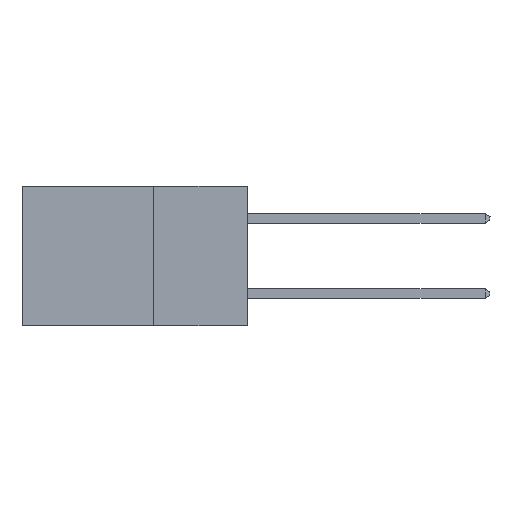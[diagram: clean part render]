
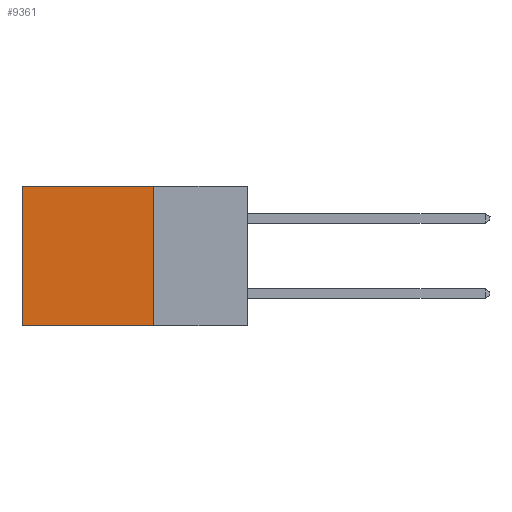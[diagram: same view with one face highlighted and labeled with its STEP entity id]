
A CAD part, left-side view. The second image highlights one B-rep face of the part: STEP entity #9361.
In plain terms, the highlighted planar face has unit normal (-1, 0, 0).
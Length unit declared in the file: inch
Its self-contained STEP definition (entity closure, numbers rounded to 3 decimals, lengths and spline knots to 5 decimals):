
#234 = CARTESIAN_POINT ( 'NONE',  ( 0.298, 0.6, 0. ) ) ;
#791 = VECTOR ( 'NONE', #5980, 39.37008 ) ;
#3077 = DIRECTION ( 'NONE',  ( 1., 0., 0. ) ) ;
#3121 = EDGE_CURVE ( 'NONE', #14947, #22055, #24953, .T. ) ;
#4579 = EDGE_CURVE ( 'NONE', #10231, #8371, #10458, .T. ) ;
#4825 = ORIENTED_EDGE ( 'NONE', *, *, #10721, .F. ) ;
#5660 = CARTESIAN_POINT ( 'NONE',  ( 0.298, 0.6, -0.37 ) ) ;
#5980 = DIRECTION ( 'NONE',  ( 0., 0., -1. ) ) ;
#6827 = VECTOR ( 'NONE', #19081, 39.37008 ) ;
#7606 = EDGE_LOOP ( 'NONE', ( #22664, #16860, #4825, #17059 ) ) ;
#8371 = VERTEX_POINT ( 'NONE', #23700 ) ;
#8498 = VECTOR ( 'NONE', #12989, 39.37008 ) ;
#9361 = ADVANCED_FACE ( 'NONE', ( #17837 ), #17186, .F. ) ;
#10231 = VERTEX_POINT ( 'NONE', #25343 ) ;
#10458 = LINE ( 'NONE', #19895, #18463 ) ;
#10721 = EDGE_CURVE ( 'NONE', #10231, #14947, #19887, .T. ) ;
#12240 = DIRECTION ( 'NONE',  ( 0., 1., 0. ) ) ;
#12634 = CARTESIAN_POINT ( 'NONE',  ( 0.298, 0.25, 0. ) ) ;
#12989 = DIRECTION ( 'NONE',  ( 0., 0., -1. ) ) ;
#13406 = CARTESIAN_POINT ( 'NONE',  ( 0.298, 0.25, -0.37 ) ) ;
#13700 = AXIS2_PLACEMENT_3D ( 'NONE', #24721, #3077, #18837 ) ;
#14947 = VERTEX_POINT ( 'NONE', #17320 ) ;
#16860 = ORIENTED_EDGE ( 'NONE', *, *, #3121, .F. ) ;
#17059 = ORIENTED_EDGE ( 'NONE', *, *, #4579, .T. ) ;
#17186 = PLANE ( 'NONE',  #13700 ) ;
#17320 = CARTESIAN_POINT ( 'NONE',  ( 0.298, 0.25, -0.37 ) ) ;
#17837 = FACE_OUTER_BOUND ( 'NONE', #7606, .T. ) ;
#18463 = VECTOR ( 'NONE', #12240, 39.37008 ) ;
#18837 = DIRECTION ( 'NONE',  ( 0., 0., -1. ) ) ;
#19024 = LINE ( 'NONE', #234, #791 ) ;
#19081 = DIRECTION ( 'NONE',  ( 0., 1., 0. ) ) ;
#19887 = LINE ( 'NONE', #12634, #8498 ) ;
#19895 = CARTESIAN_POINT ( 'NONE',  ( 0.298, 0.25, 0. ) ) ;
#22055 = VERTEX_POINT ( 'NONE', #5660 ) ;
#22664 = ORIENTED_EDGE ( 'NONE', *, *, #24938, .T. ) ;
#23700 = CARTESIAN_POINT ( 'NONE',  ( 0.298, 0.6, 0. ) ) ;
#24721 = CARTESIAN_POINT ( 'NONE',  ( 0.298, 0.25, 0. ) ) ;
#24938 = EDGE_CURVE ( 'NONE', #8371, #22055, #19024, .T. ) ;
#24953 = LINE ( 'NONE', #13406, #6827 ) ;
#25343 = CARTESIAN_POINT ( 'NONE',  ( 0.298, 0.25, 0. ) ) ;
